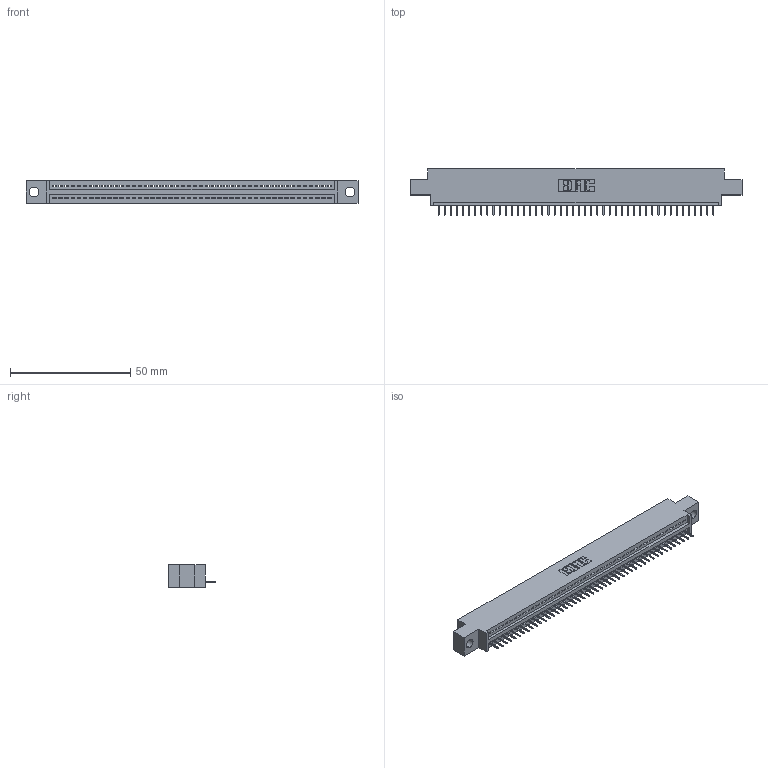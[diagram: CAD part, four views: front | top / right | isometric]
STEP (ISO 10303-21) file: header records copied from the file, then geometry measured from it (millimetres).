
FILE_DESCRIPTION (( 'STEP AP203' ), '1' );
FILE_NAME ('345-046-524-604.STEP', '2021-05-26T15:11:18', ( '' ), ( '' ), 'SwSTEP 2.0', 'SolidWorks 2020', '' );
FILE_SCHEMA (( 'CONFIG_CONTROL_DESIGN' ));
Length unit declared in the file: inch
Products named in the file (3): 345-046-524-604; 345-292-001_345-293-124; 345 Part_0.170 Offset - 0.156 Dia-TI
Assembly tree (47 placements, depth 2):
  345-046-524-604
    345 Part_0.170 Offset - 0.156 Dia-TI
    345-292-001_345-293-124  x46
Bounding box: 138.05 x 19.35 x 9.4 mm (x, y, z)
Volume: 12743.8 mm3; surface area: 16377.7 mm2
Topology: 47 solids, 47 shells, 2996 faces, 8669 edges, 5594 vertices
Faces by surface type: plane 2214, cylinder 782
Entity records: 34707 total; most frequent: CARTESIAN_POINT 6020, ORIENTED_EDGE 5998, DIRECTION 5251, EDGE_CURVE 2999, LINE 2687, VECTOR 2687, VERTEX_POINT 1994, AXIS2_PLACEMENT_3D 1282
